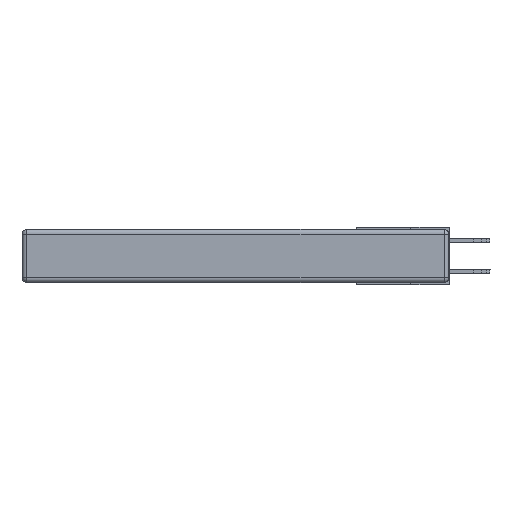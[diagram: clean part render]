
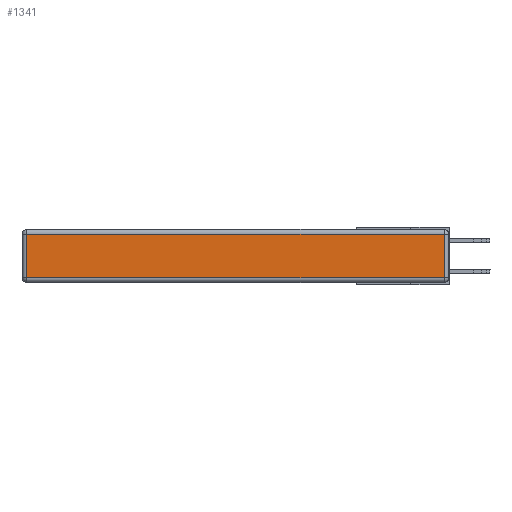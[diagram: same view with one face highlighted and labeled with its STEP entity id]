
A CAD part, left-side view. The second image highlights one B-rep face of the part: STEP entity #1341.
In plain terms, the highlighted planar face has unit normal (-1, 0, 0).
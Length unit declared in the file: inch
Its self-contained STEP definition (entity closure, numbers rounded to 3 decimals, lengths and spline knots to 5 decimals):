
#53 = CARTESIAN_POINT ( 'NONE',  ( 0., 2.75, -0.03 ) ) ;
#629 = ORIENTED_EDGE ( 'NONE', *, *, #14416, .T. ) ;
#1341 = ADVANCED_FACE ( 'NONE', ( #10687 ), #2610, .T. ) ;
#1914 = DIRECTION ( 'NONE',  ( 0., 0., -1. ) ) ;
#2412 = VERTEX_POINT ( 'NONE', #14765 ) ;
#2610 = PLANE ( 'NONE',  #13766 ) ;
#2896 = VECTOR ( 'NONE', #10627, 39.37008 ) ;
#3180 = CARTESIAN_POINT ( 'NONE',  ( 0., 0.03, -0.03 ) ) ;
#4166 = VERTEX_POINT ( 'NONE', #3180 ) ;
#4499 = VERTEX_POINT ( 'NONE', #10486 ) ;
#4521 = VECTOR ( 'NONE', #11033, 39.37008 ) ;
#5882 = VECTOR ( 'NONE', #1914, 39.37008 ) ;
#6847 = DIRECTION ( 'NONE',  ( 0., 0., 1. ) ) ;
#7289 = ORIENTED_EDGE ( 'NONE', *, *, #11594, .T. ) ;
#7330 = LINE ( 'NONE', #17625, #12956 ) ;
#7425 = LINE ( 'NONE', #12208, #2896 ) ;
#7723 = ORIENTED_EDGE ( 'NONE', *, *, #14376, .T. ) ;
#7926 = ORIENTED_EDGE ( 'NONE', *, *, #12309, .T. ) ;
#9438 = CARTESIAN_POINT ( 'NONE',  ( 0., 0., -0.343 ) ) ;
#10288 = CARTESIAN_POINT ( 'NONE',  ( 0., 2.72, -0.343 ) ) ;
#10486 = CARTESIAN_POINT ( 'NONE',  ( 0., 2.72, -0.313 ) ) ;
#10587 = LINE ( 'NONE', #53, #4521 ) ;
#10627 = DIRECTION ( 'NONE',  ( 0., -1., 0. ) ) ;
#10687 = FACE_OUTER_BOUND ( 'NONE', #13252, .T. ) ;
#11033 = DIRECTION ( 'NONE',  ( 0., 1., 0. ) ) ;
#11594 = EDGE_CURVE ( 'NONE', #4499, #2412, #7425, .T. ) ;
#12208 = CARTESIAN_POINT ( 'NONE',  ( 0., 0., -0.313 ) ) ;
#12309 = EDGE_CURVE ( 'NONE', #17494, #4499, #13669, .T. ) ;
#12956 = VECTOR ( 'NONE', #6847, 39.37008 ) ;
#13009 = CARTESIAN_POINT ( 'NONE',  ( 0., 2.72, -0.03 ) ) ;
#13252 = EDGE_LOOP ( 'NONE', ( #7289, #7723, #629, #7926 ) ) ;
#13669 = LINE ( 'NONE', #10288, #5882 ) ;
#13766 = AXIS2_PLACEMENT_3D ( 'NONE', #9438, #17607, #14907 ) ;
#14376 = EDGE_CURVE ( 'NONE', #2412, #4166, #7330, .T. ) ;
#14416 = EDGE_CURVE ( 'NONE', #4166, #17494, #10587, .T. ) ;
#14765 = CARTESIAN_POINT ( 'NONE',  ( 0., 0.03, -0.313 ) ) ;
#14907 = DIRECTION ( 'NONE',  ( 0., 0., 1. ) ) ;
#17494 = VERTEX_POINT ( 'NONE', #13009 ) ;
#17607 = DIRECTION ( 'NONE',  ( -1., 0., 0. ) ) ;
#17625 = CARTESIAN_POINT ( 'NONE',  ( 0., 0.03, -0.343 ) ) ;
